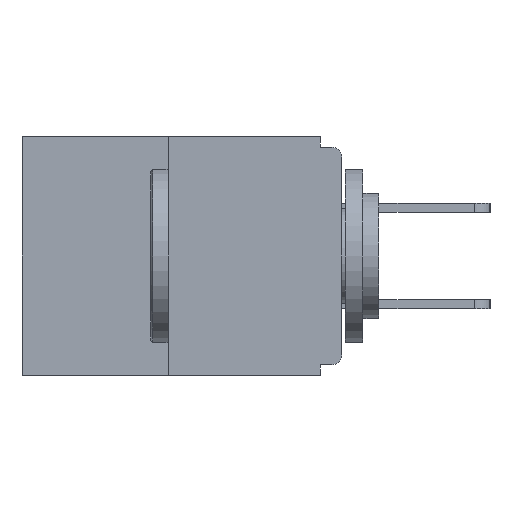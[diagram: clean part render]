
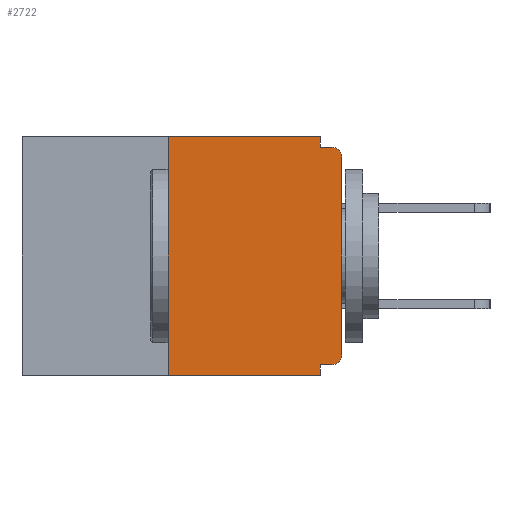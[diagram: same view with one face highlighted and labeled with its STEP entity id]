
A CAD part, left-side view. The second image highlights one B-rep face of the part: STEP entity #2722.
In plain terms, the highlighted planar face has unit normal (-1, 0, 0).
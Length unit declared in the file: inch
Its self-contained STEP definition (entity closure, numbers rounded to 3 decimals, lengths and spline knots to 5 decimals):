
#77 = VERTEX_POINT ( 'NONE', #1014 ) ;
#681 = EDGE_CURVE ( 'NONE', #13280, #9607, #11232, .T. ) ;
#777 = CARTESIAN_POINT ( 'NONE',  ( 0., 0.031, -0.015 ) ) ;
#896 = AXIS2_PLACEMENT_3D ( 'NONE', #1206, #11165, #3535 ) ;
#916 = VERTEX_POINT ( 'NONE', #10670 ) ;
#985 = EDGE_CURVE ( 'NONE', #3789, #916, #12454, .T. ) ;
#1014 = CARTESIAN_POINT ( 'NONE',  ( 0., 0.015, -0.015 ) ) ;
#1206 = CARTESIAN_POINT ( 'NONE',  ( 0., 0.015, -0.03 ) ) ;
#1236 = CARTESIAN_POINT ( 'NONE',  ( 0., 0.46, 0. ) ) ;
#1668 = DIRECTION ( 'NONE',  ( 0., 0., -1. ) ) ;
#1746 = EDGE_CURVE ( 'NONE', #3789, #8437, #4588, .T. ) ;
#1816 = VECTOR ( 'NONE', #14707, 39.37008 ) ;
#2149 = CARTESIAN_POINT ( 'NONE',  ( 0., 0.015, -0.328 ) ) ;
#2520 = CARTESIAN_POINT ( 'NONE',  ( 0., 0.46, 0. ) ) ;
#2722 = ADVANCED_FACE ( 'NONE', ( #10779 ), #6273, .F. ) ;
#2758 = CARTESIAN_POINT ( 'NONE',  ( 0., 0., -0.328 ) ) ;
#2952 = VECTOR ( 'NONE', #7735, 39.37008 ) ;
#3288 = LINE ( 'NONE', #8900, #10261 ) ;
#3535 = DIRECTION ( 'NONE',  ( 0., 0., -1. ) ) ;
#3643 = DIRECTION ( 'NONE',  ( 0., 0., 1. ) ) ;
#3702 = EDGE_CURVE ( 'NONE', #916, #12854, #9143, .T. ) ;
#3789 = VERTEX_POINT ( 'NONE', #2149 ) ;
#3860 = DIRECTION ( 'NONE',  ( 1., 0., 0. ) ) ;
#3870 = CARTESIAN_POINT ( 'NONE',  ( 0., 0.031, -0.328 ) ) ;
#4418 = VECTOR ( 'NONE', #11489, 39.37008 ) ;
#4588 = LINE ( 'NONE', #2758, #6753 ) ;
#4698 = ORIENTED_EDGE ( 'NONE', *, *, #1746, .F. ) ;
#4995 = CARTESIAN_POINT ( 'NONE',  ( 0., 0.25, 0. ) ) ;
#5218 = CARTESIAN_POINT ( 'NONE',  ( 0., 0.25, 0. ) ) ;
#5253 = VERTEX_POINT ( 'NONE', #5218 ) ;
#5339 = DIRECTION ( 'NONE',  ( 0., 1., 0. ) ) ;
#5493 = CARTESIAN_POINT ( 'NONE',  ( 0., 0.031, -0.343 ) ) ;
#5610 = DIRECTION ( 'NONE',  ( 0., 0., -1. ) ) ;
#5619 = AXIS2_PLACEMENT_3D ( 'NONE', #7293, #9993, #15107 ) ;
#5628 = CIRCLE ( 'NONE', #896, 0.015 ) ;
#6006 = ORIENTED_EDGE ( 'NONE', *, *, #9776, .F. ) ;
#6171 = EDGE_CURVE ( 'NONE', #16084, #77, #3288, .T. ) ;
#6273 = PLANE ( 'NONE',  #16017 ) ;
#6358 = CARTESIAN_POINT ( 'NONE',  ( 0., 0.031, 0. ) ) ;
#6734 = CARTESIAN_POINT ( 'NONE',  ( 0., 0., -0.03 ) ) ;
#6753 = VECTOR ( 'NONE', #5339, 39.37008 ) ;
#6953 = ORIENTED_EDGE ( 'NONE', *, *, #3702, .T. ) ;
#7293 = CARTESIAN_POINT ( 'NONE',  ( 0., 0.015, -0.313 ) ) ;
#7735 = DIRECTION ( 'NONE',  ( 0., 0., 1. ) ) ;
#8060 = ORIENTED_EDGE ( 'NONE', *, *, #985, .T. ) ;
#8336 = ORIENTED_EDGE ( 'NONE', *, *, #15807, .F. ) ;
#8437 = VERTEX_POINT ( 'NONE', #3870 ) ;
#8900 = CARTESIAN_POINT ( 'NONE',  ( 0., 0., -0.015 ) ) ;
#8973 = CARTESIAN_POINT ( 'NONE',  ( 0., 0., 0. ) ) ;
#9063 = ORIENTED_EDGE ( 'NONE', *, *, #681, .T. ) ;
#9143 = LINE ( 'NONE', #8973, #2952 ) ;
#9607 = VERTEX_POINT ( 'NONE', #5493 ) ;
#9776 = EDGE_CURVE ( 'NONE', #13280, #5253, #11811, .T. ) ;
#9908 = EDGE_LOOP ( 'NONE', ( #14421, #6006, #9063, #11976, #4698, #8060, #6953, #16024, #15296, #8336 ) ) ;
#9924 = EDGE_CURVE ( 'NONE', #12854, #77, #5628, .T. ) ;
#9993 = DIRECTION ( 'NONE',  ( -1., 0., 0. ) ) ;
#10261 = VECTOR ( 'NONE', #11536, 39.37008 ) ;
#10670 = CARTESIAN_POINT ( 'NONE',  ( 0., 0., -0.313 ) ) ;
#10779 = FACE_OUTER_BOUND ( 'NONE', #9908, .T. ) ;
#11165 = DIRECTION ( 'NONE',  ( -1., 0., 0. ) ) ;
#11232 = LINE ( 'NONE', #16126, #1816 ) ;
#11489 = DIRECTION ( 'NONE',  ( 0., -1., 0. ) ) ;
#11536 = DIRECTION ( 'NONE',  ( 0., -1., 0. ) ) ;
#11543 = LINE ( 'NONE', #6358, #14988 ) ;
#11596 = CARTESIAN_POINT ( 'NONE',  ( 0., 0.25, -0.343 ) ) ;
#11811 = LINE ( 'NONE', #4995, #13237 ) ;
#11976 = ORIENTED_EDGE ( 'NONE', *, *, #14699, .F. ) ;
#12039 = VERTEX_POINT ( 'NONE', #15098 ) ;
#12454 = CIRCLE ( 'NONE', #5619, 0.015 ) ;
#12854 = VERTEX_POINT ( 'NONE', #6734 ) ;
#13237 = VECTOR ( 'NONE', #3643, 39.37008 ) ;
#13280 = VERTEX_POINT ( 'NONE', #11596 ) ;
#14112 = EDGE_CURVE ( 'NONE', #5253, #12039, #15234, .T. ) ;
#14421 = ORIENTED_EDGE ( 'NONE', *, *, #14112, .F. ) ;
#14440 = LINE ( 'NONE', #15920, #15838 ) ;
#14699 = EDGE_CURVE ( 'NONE', #8437, #9607, #14440, .T. ) ;
#14707 = DIRECTION ( 'NONE',  ( 0., -1., 0. ) ) ;
#14988 = VECTOR ( 'NONE', #1668, 39.37008 ) ;
#15098 = CARTESIAN_POINT ( 'NONE',  ( 0., 0.031, 0. ) ) ;
#15107 = DIRECTION ( 'NONE',  ( 0., 0., -1. ) ) ;
#15234 = LINE ( 'NONE', #2520, #4418 ) ;
#15296 = ORIENTED_EDGE ( 'NONE', *, *, #6171, .F. ) ;
#15395 = DIRECTION ( 'NONE',  ( 0., 0., -1. ) ) ;
#15807 = EDGE_CURVE ( 'NONE', #12039, #16084, #11543, .T. ) ;
#15838 = VECTOR ( 'NONE', #5610, 39.37008 ) ;
#15920 = CARTESIAN_POINT ( 'NONE',  ( 0., 0.031, -0.343 ) ) ;
#16017 = AXIS2_PLACEMENT_3D ( 'NONE', #1236, #3860, #15395 ) ;
#16024 = ORIENTED_EDGE ( 'NONE', *, *, #9924, .T. ) ;
#16084 = VERTEX_POINT ( 'NONE', #777 ) ;
#16126 = CARTESIAN_POINT ( 'NONE',  ( 0., 0.46, -0.343 ) ) ;
